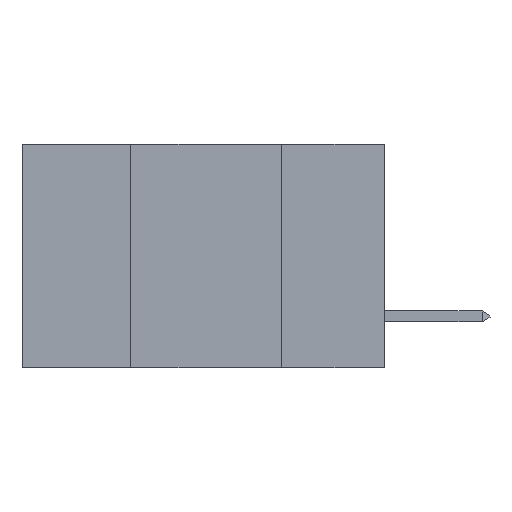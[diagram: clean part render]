
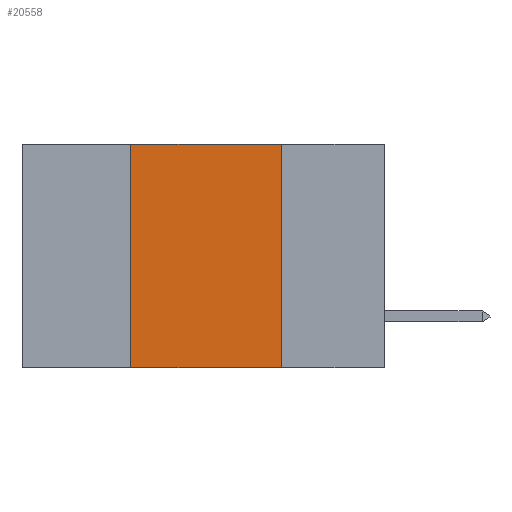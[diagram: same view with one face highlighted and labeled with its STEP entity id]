
A CAD part, left-side view. The second image highlights one B-rep face of the part: STEP entity #20558.
In plain terms, the highlighted planar face has unit normal (-1, 0, 0).
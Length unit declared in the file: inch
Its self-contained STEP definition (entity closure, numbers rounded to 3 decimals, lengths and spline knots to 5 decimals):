
#31 = VERTEX_POINT ( 'NONE', #3668 ) ;
#543 = FACE_OUTER_BOUND ( 'NONE', #9704, .T. ) ;
#1563 = EDGE_CURVE ( 'NONE', #10090, #14368, #17040, .T. ) ;
#2345 = VECTOR ( 'NONE', #7161, 39.37008 ) ;
#3005 = EDGE_CURVE ( 'NONE', #10090, #31, #26118, .T. ) ;
#3608 = CARTESIAN_POINT ( 'NONE',  ( 0., 0.42, -0.37 ) ) ;
#3668 = CARTESIAN_POINT ( 'NONE',  ( 0., 0.42, 0. ) ) ;
#3673 = VERTEX_POINT ( 'NONE', #20511 ) ;
#4421 = EDGE_CURVE ( 'NONE', #3673, #14368, #19395, .T. ) ;
#5260 = CARTESIAN_POINT ( 'NONE',  ( 0., 0.17, 0. ) ) ;
#6143 = VECTOR ( 'NONE', #17254, 39.37008 ) ;
#7161 = DIRECTION ( 'NONE',  ( 0., -1., 0. ) ) ;
#8848 = AXIS2_PLACEMENT_3D ( 'NONE', #23043, #11107, #24998 ) ;
#9704 = EDGE_LOOP ( 'NONE', ( #16278, #22435, #21998, #21025 ) ) ;
#10090 = VERTEX_POINT ( 'NONE', #3608 ) ;
#11107 = DIRECTION ( 'NONE',  ( 1., 0., 0. ) ) ;
#13093 = PLANE ( 'NONE',  #8848 ) ;
#13840 = EDGE_CURVE ( 'NONE', #31, #3673, #23950, .T. ) ;
#14368 = VERTEX_POINT ( 'NONE', #15016 ) ;
#15016 = CARTESIAN_POINT ( 'NONE',  ( 0., 0.17, -0.37 ) ) ;
#15686 = VECTOR ( 'NONE', #19628, 39.37008 ) ;
#16278 = ORIENTED_EDGE ( 'NONE', *, *, #4421, .F. ) ;
#17040 = LINE ( 'NONE', #21214, #6143 ) ;
#17254 = DIRECTION ( 'NONE',  ( 0., -1., 0. ) ) ;
#19395 = LINE ( 'NONE', #5260, #24547 ) ;
#19628 = DIRECTION ( 'NONE',  ( 0., 0., 1. ) ) ;
#20511 = CARTESIAN_POINT ( 'NONE',  ( 0., 0.17, 0. ) ) ;
#20558 = ADVANCED_FACE ( 'NONE', ( #543 ), #13093, .F. ) ;
#21025 = ORIENTED_EDGE ( 'NONE', *, *, #1563, .T. ) ;
#21214 = CARTESIAN_POINT ( 'NONE',  ( 0., 0.6, -0.37 ) ) ;
#21998 = ORIENTED_EDGE ( 'NONE', *, *, #3005, .F. ) ;
#22435 = ORIENTED_EDGE ( 'NONE', *, *, #13840, .F. ) ;
#23043 = CARTESIAN_POINT ( 'NONE',  ( 0., 0.6, 0. ) ) ;
#23242 = CARTESIAN_POINT ( 'NONE',  ( 0., 0.6, 0. ) ) ;
#23435 = CARTESIAN_POINT ( 'NONE',  ( 0., 0.42, 0. ) ) ;
#23950 = LINE ( 'NONE', #23242, #2345 ) ;
#24547 = VECTOR ( 'NONE', #24700, 39.37008 ) ;
#24700 = DIRECTION ( 'NONE',  ( 0., 0., -1. ) ) ;
#24998 = DIRECTION ( 'NONE',  ( 0., 0., -1. ) ) ;
#26118 = LINE ( 'NONE', #23435, #15686 ) ;
